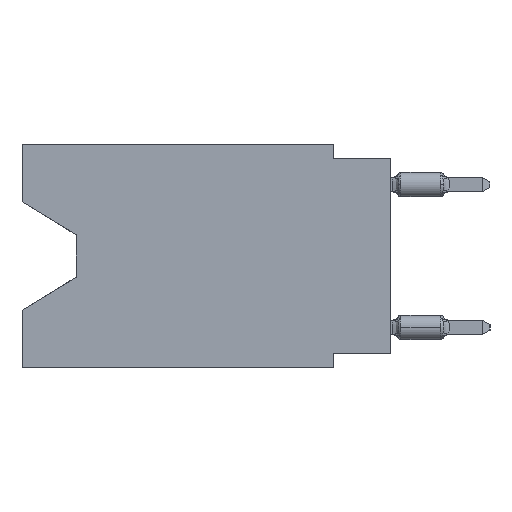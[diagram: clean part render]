
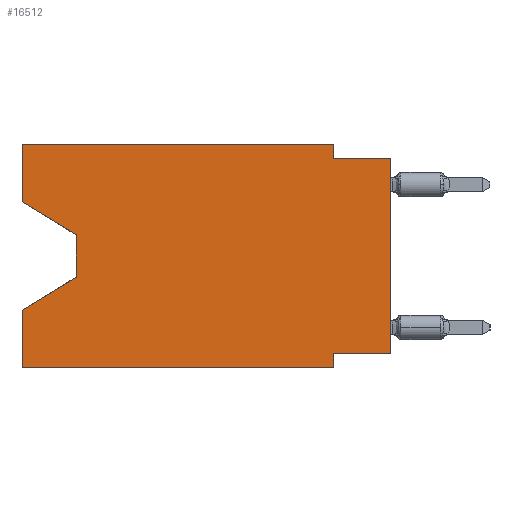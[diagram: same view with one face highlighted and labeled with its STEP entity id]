
A CAD part, left-side view. The second image highlights one B-rep face of the part: STEP entity #16512.
In plain terms, the highlighted planar face has unit normal (-1, 0, 0).
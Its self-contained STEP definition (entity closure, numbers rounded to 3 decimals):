
#544 = VERTEX_POINT ( 'NONE', #47119 ) ;
#780 = VECTOR ( 'NONE', #20437, 1000. ) ;
#3247 = CARTESIAN_POINT ( 'NONE',  ( 0., 2.54, -9.906 ) ) ;
#3406 = LINE ( 'NONE', #43582, #3703 ) ;
#3703 = VECTOR ( 'NONE', #59688, 1000. ) ;
#3885 = EDGE_CURVE ( 'NONE', #43309, #25918, #32214, .T. ) ;
#4143 = CARTESIAN_POINT ( 'NONE',  ( 0., 16.383, 0. ) ) ;
#5637 = CARTESIAN_POINT ( 'NONE',  ( 0., 13.97, -4.013 ) ) ;
#5854 = EDGE_CURVE ( 'NONE', #51954, #9394, #60923, .T. ) ;
#5962 = LINE ( 'NONE', #5637, #35472 ) ;
#7063 = CARTESIAN_POINT ( 'NONE',  ( 0., 2.54, -9.271 ) ) ;
#8081 = EDGE_CURVE ( 'NONE', #26708, #25918, #11228, .T. ) ;
#9394 = VERTEX_POINT ( 'NONE', #58523 ) ;
#9784 = EDGE_CURVE ( 'NONE', #9394, #26708, #3406, .T. ) ;
#9945 = VERTEX_POINT ( 'NONE', #10410 ) ;
#10410 = CARTESIAN_POINT ( 'NONE',  ( 0., 16.383, -2.546 ) ) ;
#11228 = LINE ( 'NONE', #27574, #22665 ) ;
#11323 = DIRECTION ( 'NONE',  ( 0., 0., -1. ) ) ;
#11349 = DIRECTION ( 'NONE',  ( 0., 0., 1. ) ) ;
#11761 = VECTOR ( 'NONE', #15331, 1000. ) ;
#11941 = ORIENTED_EDGE ( 'NONE', *, *, #53324, .T. ) ;
#12010 = VECTOR ( 'NONE', #14536, 1000. ) ;
#14409 = LINE ( 'NONE', #49906, #23060 ) ;
#14536 = DIRECTION ( 'NONE',  ( 0., 0., 1. ) ) ;
#14880 = VERTEX_POINT ( 'NONE', #7063 ) ;
#14958 = CARTESIAN_POINT ( 'NONE',  ( 0., 0., -0.635 ) ) ;
#15290 = VECTOR ( 'NONE', #63886, 1000. ) ;
#15331 = DIRECTION ( 'NONE',  ( 0., -1., 0. ) ) ;
#16241 = VERTEX_POINT ( 'NONE', #51427 ) ;
#16512 = ADVANCED_FACE ( 'NONE', ( #50025 ), #19203, .F. ) ;
#16842 = ORIENTED_EDGE ( 'NONE', *, *, #65614, .T. ) ;
#18554 = LINE ( 'NONE', #65164, #12010 ) ;
#18865 = DIRECTION ( 'NONE',  ( 0., 0., -1. ) ) ;
#19203 = PLANE ( 'NONE',  #29679 ) ;
#20437 = DIRECTION ( 'NONE',  ( 0., 1., 0. ) ) ;
#20855 = EDGE_CURVE ( 'NONE', #16241, #41680, #5962, .T. ) ;
#22665 = VECTOR ( 'NONE', #57793, 1000. ) ;
#23060 = VECTOR ( 'NONE', #24754, 1000. ) ;
#23348 = EDGE_CURVE ( 'NONE', #9945, #51954, #18554, .T. ) ;
#23889 = DIRECTION ( 'NONE',  ( 1., 0., 0. ) ) ;
#24220 = CARTESIAN_POINT ( 'NONE',  ( 0., 13.97, -5.893 ) ) ;
#24448 = DIRECTION ( 'NONE',  ( 0., 0., 1. ) ) ;
#24754 = DIRECTION ( 'NONE',  ( 0., 0., -1. ) ) ;
#25104 = LINE ( 'NONE', #49936, #780 ) ;
#25314 = ORIENTED_EDGE ( 'NONE', *, *, #26615, .F. ) ;
#25635 = VECTOR ( 'NONE', #24448, 1000. ) ;
#25722 = CARTESIAN_POINT ( 'NONE',  ( 0., 16.383, -9.906 ) ) ;
#25918 = VERTEX_POINT ( 'NONE', #14958 ) ;
#26615 = EDGE_CURVE ( 'NONE', #14880, #34806, #14409, .T. ) ;
#26708 = VERTEX_POINT ( 'NONE', #50568 ) ;
#27574 = CARTESIAN_POINT ( 'NONE',  ( 0., 0., -0.635 ) ) ;
#28266 = EDGE_CURVE ( 'NONE', #43309, #14880, #25104, .T. ) ;
#28451 = VECTOR ( 'NONE', #64983, 1000. ) ;
#28587 = ORIENTED_EDGE ( 'NONE', *, *, #23348, .F. ) ;
#29440 = ORIENTED_EDGE ( 'NONE', *, *, #3885, .T. ) ;
#29679 = AXIS2_PLACEMENT_3D ( 'NONE', #4143, #23889, #18865 ) ;
#30158 = VECTOR ( 'NONE', #33494, 1000. ) ;
#31201 = ORIENTED_EDGE ( 'NONE', *, *, #5854, .F. ) ;
#32214 = LINE ( 'NONE', #52669, #25635 ) ;
#32583 = ORIENTED_EDGE ( 'NONE', *, *, #58794, .T. ) ;
#33494 = DIRECTION ( 'NONE',  ( 0., 0.855, -0.519 ) ) ;
#34806 = VERTEX_POINT ( 'NONE', #3247 ) ;
#35437 = CARTESIAN_POINT ( 'NONE',  ( 0., 16.383, 0. ) ) ;
#35472 = VECTOR ( 'NONE', #11323, 1000. ) ;
#36635 = ORIENTED_EDGE ( 'NONE', *, *, #28266, .F. ) ;
#38017 = EDGE_LOOP ( 'NONE', ( #32583, #60900, #16842, #56023, #11941, #25314, #36635, #29440, #45093, #65999, #31201, #28587 ) ) ;
#38515 = CARTESIAN_POINT ( 'NONE',  ( 0., 13.97, -5.893 ) ) ;
#41680 = VERTEX_POINT ( 'NONE', #24220 ) ;
#43309 = VERTEX_POINT ( 'NONE', #61147 ) ;
#43582 = CARTESIAN_POINT ( 'NONE',  ( 0., 2.54, 0. ) ) ;
#44414 = LINE ( 'NONE', #64889, #15290 ) ;
#45093 = ORIENTED_EDGE ( 'NONE', *, *, #8081, .F. ) ;
#45844 = CARTESIAN_POINT ( 'NONE',  ( 0., 16.383, -2.546 ) ) ;
#47119 = CARTESIAN_POINT ( 'NONE',  ( 0., 16.383, -7.36 ) ) ;
#49906 = CARTESIAN_POINT ( 'NONE',  ( 0., 2.54, -9.906 ) ) ;
#49936 = CARTESIAN_POINT ( 'NONE',  ( 0., 0., -9.271 ) ) ;
#50025 = FACE_OUTER_BOUND ( 'NONE', #38017, .T. ) ;
#50568 = CARTESIAN_POINT ( 'NONE',  ( 0., 2.54, -0.635 ) ) ;
#50627 = VERTEX_POINT ( 'NONE', #25722 ) ;
#51189 = LINE ( 'NONE', #45844, #28451 ) ;
#51427 = CARTESIAN_POINT ( 'NONE',  ( 0., 13.97, -4.013 ) ) ;
#51954 = VERTEX_POINT ( 'NONE', #57870 ) ;
#52210 = LINE ( 'NONE', #57252, #65406 ) ;
#52669 = CARTESIAN_POINT ( 'NONE',  ( 0., 0., 0. ) ) ;
#53324 = EDGE_CURVE ( 'NONE', #50627, #34806, #44414, .T. ) ;
#56023 = ORIENTED_EDGE ( 'NONE', *, *, #64129, .F. ) ;
#57252 = CARTESIAN_POINT ( 'NONE',  ( 0., 16.383, 0. ) ) ;
#57793 = DIRECTION ( 'NONE',  ( 0., -1., 0. ) ) ;
#57870 = CARTESIAN_POINT ( 'NONE',  ( 0., 16.383, 0. ) ) ;
#58523 = CARTESIAN_POINT ( 'NONE',  ( 0., 2.54, 0. ) ) ;
#58794 = EDGE_CURVE ( 'NONE', #9945, #16241, #51189, .T. ) ;
#59688 = DIRECTION ( 'NONE',  ( 0., 0., -1. ) ) ;
#60900 = ORIENTED_EDGE ( 'NONE', *, *, #20855, .T. ) ;
#60923 = LINE ( 'NONE', #35437, #11761 ) ;
#61147 = CARTESIAN_POINT ( 'NONE',  ( 0., 0., -9.271 ) ) ;
#63886 = DIRECTION ( 'NONE',  ( 0., -1., 0. ) ) ;
#64006 = LINE ( 'NONE', #38515, #30158 ) ;
#64129 = EDGE_CURVE ( 'NONE', #50627, #544, #52210, .T. ) ;
#64889 = CARTESIAN_POINT ( 'NONE',  ( 0., 16.383, -9.906 ) ) ;
#64983 = DIRECTION ( 'NONE',  ( 0., -0.855, -0.519 ) ) ;
#65164 = CARTESIAN_POINT ( 'NONE',  ( 0., 16.383, 0. ) ) ;
#65406 = VECTOR ( 'NONE', #11349, 1000. ) ;
#65614 = EDGE_CURVE ( 'NONE', #41680, #544, #64006, .T. ) ;
#65999 = ORIENTED_EDGE ( 'NONE', *, *, #9784, .F. ) ;
